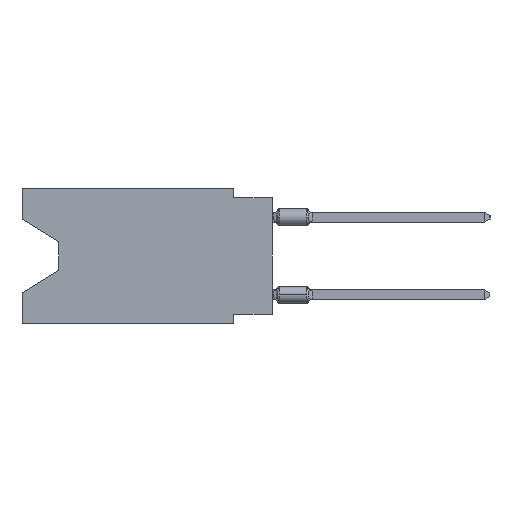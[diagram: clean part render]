
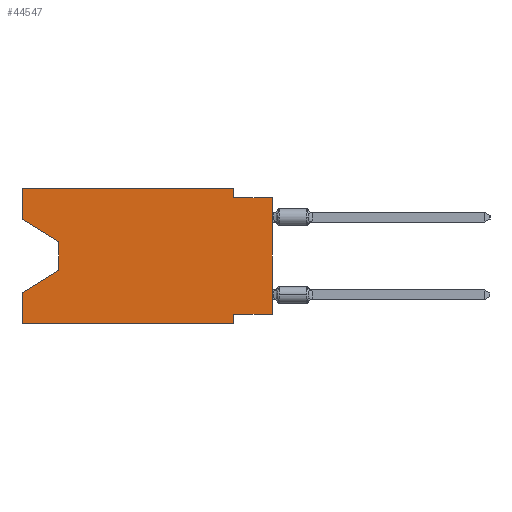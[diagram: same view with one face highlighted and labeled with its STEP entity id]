
A CAD part, left-side view. The second image highlights one B-rep face of the part: STEP entity #44547.
In plain terms, the highlighted planar face has unit normal (-1, 0, 0).
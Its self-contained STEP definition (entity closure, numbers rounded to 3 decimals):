
#38 = CARTESIAN_POINT ( 'NONE',  ( 0., 13.97, -3.505 ) ) ;
#365 = VECTOR ( 'NONE', #48831, 1000. ) ;
#1304 = CARTESIAN_POINT ( 'NONE',  ( 0., 2.54, -8.89 ) ) ;
#1531 = FACE_OUTER_BOUND ( 'NONE', #18524, .T. ) ;
#2863 = CARTESIAN_POINT ( 'NONE',  ( 0., 2.54, 0. ) ) ;
#2929 = CARTESIAN_POINT ( 'NONE',  ( 0., 0., -0.635 ) ) ;
#3101 = VECTOR ( 'NONE', #38248, 1000. ) ;
#3471 = CARTESIAN_POINT ( 'NONE',  ( 0., 16.383, -8.89 ) ) ;
#3764 = EDGE_CURVE ( 'NONE', #26340, #34917, #22129, .T. ) ;
#4080 = EDGE_CURVE ( 'NONE', #44885, #10114, #24765, .T. ) ;
#4369 = CARTESIAN_POINT ( 'NONE',  ( 0., 16.383, -8.89 ) ) ;
#4925 = CARTESIAN_POINT ( 'NONE',  ( 0., 16.383, 0. ) ) ;
#5095 = EDGE_CURVE ( 'NONE', #10114, #45868, #31322, .T. ) ;
#5727 = VECTOR ( 'NONE', #48440, 1000. ) ;
#6338 = CARTESIAN_POINT ( 'NONE',  ( 0., 13.97, -3.505 ) ) ;
#6465 = DIRECTION ( 'NONE',  ( 0., 1., 0. ) ) ;
#6983 = CARTESIAN_POINT ( 'NONE',  ( 0., 13.97, -5.385 ) ) ;
#9153 = CARTESIAN_POINT ( 'NONE',  ( 0., 16.383, 0. ) ) ;
#10114 = VERTEX_POINT ( 'NONE', #38 ) ;
#10428 = EDGE_CURVE ( 'NONE', #43888, #32613, #26883, .T. ) ;
#10491 = CARTESIAN_POINT ( 'NONE',  ( 0., 0., -8.255 ) ) ;
#12284 = CARTESIAN_POINT ( 'NONE',  ( 0., 2.54, -0.635 ) ) ;
#13681 = ORIENTED_EDGE ( 'NONE', *, *, #41763, .F. ) ;
#14453 = PLANE ( 'NONE',  #18824 ) ;
#14758 = EDGE_CURVE ( 'NONE', #26340, #35330, #40296, .T. ) ;
#15702 = CARTESIAN_POINT ( 'NONE',  ( 0., 0., -8.255 ) ) ;
#16419 = CARTESIAN_POINT ( 'NONE',  ( 0., 16.383, 0. ) ) ;
#16872 = VERTEX_POINT ( 'NONE', #2929 ) ;
#18030 = DIRECTION ( 'NONE',  ( 0., 0., 1. ) ) ;
#18524 = EDGE_LOOP ( 'NONE', ( #25316, #48048, #28959, #28085, #27515, #32996, #37769, #45664, #32916, #51289, #30365, #13681 ) ) ;
#18824 = AXIS2_PLACEMENT_3D ( 'NONE', #38369, #51529, #30837 ) ;
#19765 = LINE ( 'NONE', #52532, #37849 ) ;
#19872 = DIRECTION ( 'NONE',  ( 0., -1., 0. ) ) ;
#20682 = EDGE_CURVE ( 'NONE', #32613, #35330, #50855, .T. ) ;
#22129 = LINE ( 'NONE', #4925, #3101 ) ;
#22495 = VECTOR ( 'NONE', #22639, 1000. ) ;
#22639 = DIRECTION ( 'NONE',  ( 0., 0., 1. ) ) ;
#23641 = EDGE_CURVE ( 'NONE', #53006, #45246, #46237, .T. ) ;
#24408 = EDGE_CURVE ( 'NONE', #45868, #34917, #41548, .T. ) ;
#24634 = DIRECTION ( 'NONE',  ( 0., 0.855, -0.519 ) ) ;
#24765 = LINE ( 'NONE', #36073, #5727 ) ;
#25316 = ORIENTED_EDGE ( 'NONE', *, *, #4080, .T. ) ;
#25529 = DIRECTION ( 'NONE',  ( 0., -1., 0. ) ) ;
#26340 = VERTEX_POINT ( 'NONE', #4369 ) ;
#26678 = DIRECTION ( 'NONE',  ( 0., 0., -1. ) ) ;
#26756 = VECTOR ( 'NONE', #6465, 1000. ) ;
#26883 = LINE ( 'NONE', #10491, #26756 ) ;
#27515 = ORIENTED_EDGE ( 'NONE', *, *, #14758, .T. ) ;
#28085 = ORIENTED_EDGE ( 'NONE', *, *, #3764, .F. ) ;
#28959 = ORIENTED_EDGE ( 'NONE', *, *, #24408, .T. ) ;
#29572 = LINE ( 'NONE', #49742, #32484 ) ;
#29779 = VECTOR ( 'NONE', #24634, 1000. ) ;
#30365 = ORIENTED_EDGE ( 'NONE', *, *, #23641, .F. ) ;
#30549 = CARTESIAN_POINT ( 'NONE',  ( 0., 16.383, -6.852 ) ) ;
#30837 = DIRECTION ( 'NONE',  ( 0., 0., -1. ) ) ;
#31322 = LINE ( 'NONE', #6338, #43550 ) ;
#32484 = VECTOR ( 'NONE', #18030, 1000. ) ;
#32613 = VERTEX_POINT ( 'NONE', #41065 ) ;
#32700 = LINE ( 'NONE', #2863, #365 ) ;
#32916 = ORIENTED_EDGE ( 'NONE', *, *, #52064, .F. ) ;
#32996 = ORIENTED_EDGE ( 'NONE', *, *, #20682, .F. ) ;
#33230 = CARTESIAN_POINT ( 'NONE',  ( 0., 16.383, -2.038 ) ) ;
#34826 = DIRECTION ( 'NONE',  ( 0., 0., -1. ) ) ;
#34917 = VERTEX_POINT ( 'NONE', #30549 ) ;
#34996 = LINE ( 'NONE', #43325, #22495 ) ;
#35330 = VERTEX_POINT ( 'NONE', #1304 ) ;
#36073 = CARTESIAN_POINT ( 'NONE',  ( 0., 16.383, -2.038 ) ) ;
#37769 = ORIENTED_EDGE ( 'NONE', *, *, #10428, .F. ) ;
#37849 = VECTOR ( 'NONE', #53075, 1000. ) ;
#37968 = VECTOR ( 'NONE', #26678, 1000. ) ;
#38248 = DIRECTION ( 'NONE',  ( 0., 0., 1. ) ) ;
#38369 = CARTESIAN_POINT ( 'NONE',  ( 0., 16.383, 0. ) ) ;
#39036 = EDGE_CURVE ( 'NONE', #43888, #16872, #34996, .T. ) ;
#39041 = CARTESIAN_POINT ( 'NONE',  ( 0., 2.54, -8.89 ) ) ;
#39061 = VECTOR ( 'NONE', #25529, 1000. ) ;
#40296 = LINE ( 'NONE', #3471, #48543 ) ;
#41065 = CARTESIAN_POINT ( 'NONE',  ( 0., 2.54, -8.255 ) ) ;
#41178 = EDGE_CURVE ( 'NONE', #45246, #42518, #32700, .T. ) ;
#41548 = LINE ( 'NONE', #53117, #29779 ) ;
#41742 = CARTESIAN_POINT ( 'NONE',  ( 0., 2.54, 0. ) ) ;
#41763 = EDGE_CURVE ( 'NONE', #44885, #53006, #29572, .T. ) ;
#42518 = VERTEX_POINT ( 'NONE', #12284 ) ;
#43325 = CARTESIAN_POINT ( 'NONE',  ( 0., 0., 0. ) ) ;
#43550 = VECTOR ( 'NONE', #34826, 1000. ) ;
#43888 = VERTEX_POINT ( 'NONE', #15702 ) ;
#44547 = ADVANCED_FACE ( 'NONE', ( #1531 ), #14453, .F. ) ;
#44885 = VERTEX_POINT ( 'NONE', #33230 ) ;
#45246 = VERTEX_POINT ( 'NONE', #41742 ) ;
#45664 = ORIENTED_EDGE ( 'NONE', *, *, #39036, .T. ) ;
#45868 = VERTEX_POINT ( 'NONE', #6983 ) ;
#46237 = LINE ( 'NONE', #9153, #39061 ) ;
#48048 = ORIENTED_EDGE ( 'NONE', *, *, #5095, .T. ) ;
#48440 = DIRECTION ( 'NONE',  ( 0., -0.855, -0.519 ) ) ;
#48543 = VECTOR ( 'NONE', #19872, 1000. ) ;
#48831 = DIRECTION ( 'NONE',  ( 0., 0., -1. ) ) ;
#49742 = CARTESIAN_POINT ( 'NONE',  ( 0., 16.383, 0. ) ) ;
#50855 = LINE ( 'NONE', #39041, #37968 ) ;
#51289 = ORIENTED_EDGE ( 'NONE', *, *, #41178, .F. ) ;
#51529 = DIRECTION ( 'NONE',  ( 1., 0., 0. ) ) ;
#52064 = EDGE_CURVE ( 'NONE', #42518, #16872, #19765, .T. ) ;
#52532 = CARTESIAN_POINT ( 'NONE',  ( 0., 0., -0.635 ) ) ;
#53006 = VERTEX_POINT ( 'NONE', #16419 ) ;
#53075 = DIRECTION ( 'NONE',  ( 0., -1., 0. ) ) ;
#53117 = CARTESIAN_POINT ( 'NONE',  ( 0., 13.97, -5.385 ) ) ;
